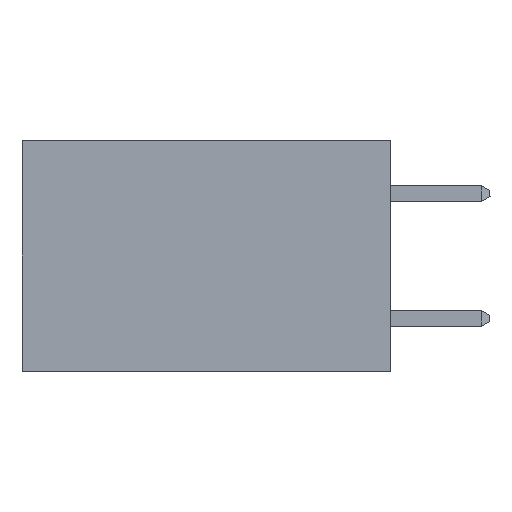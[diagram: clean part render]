
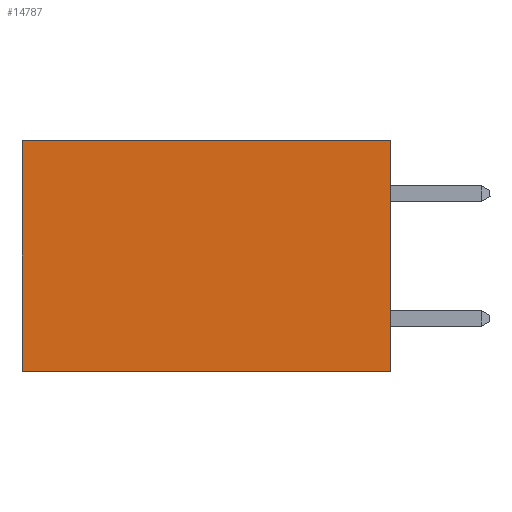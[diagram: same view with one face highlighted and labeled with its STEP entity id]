
A CAD part, left-side view. The second image highlights one B-rep face of the part: STEP entity #14787.
In plain terms, the highlighted planar face has unit normal (-1, 0, 0).
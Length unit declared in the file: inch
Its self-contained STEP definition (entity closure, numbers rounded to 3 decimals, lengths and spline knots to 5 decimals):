
#347 = CARTESIAN_POINT ( 'NONE',  ( 0.277, 0.59, 0. ) ) ;
#1477 = CARTESIAN_POINT ( 'NONE',  ( 0.277, 0., -0.37 ) ) ;
#1600 = CARTESIAN_POINT ( 'NONE',  ( 0.277, 0., -0.37 ) ) ;
#2965 = LINE ( 'NONE', #6803, #10829 ) ;
#3771 = ORIENTED_EDGE ( 'NONE', *, *, #13787, .F. ) ;
#4180 = AXIS2_PLACEMENT_3D ( 'NONE', #4374, #14548, #5916 ) ;
#4274 = FACE_OUTER_BOUND ( 'NONE', #13644, .T. ) ;
#4374 = CARTESIAN_POINT ( 'NONE',  ( 0.277, 0., -0.37 ) ) ;
#4384 = ORIENTED_EDGE ( 'NONE', *, *, #16679, .F. ) ;
#4889 = VECTOR ( 'NONE', #10450, 39.37008 ) ;
#5178 = CARTESIAN_POINT ( 'NONE',  ( 0.277, 0., 0. ) ) ;
#5480 = EDGE_CURVE ( 'NONE', #12283, #11610, #2965, .T. ) ;
#5916 = DIRECTION ( 'NONE',  ( 0., 0., -1. ) ) ;
#6198 = LINE ( 'NONE', #16697, #9669 ) ;
#6334 = ORIENTED_EDGE ( 'NONE', *, *, #15462, .T. ) ;
#6803 = CARTESIAN_POINT ( 'NONE',  ( 0.277, 0.59, -0.37 ) ) ;
#7529 = VECTOR ( 'NONE', #17961, 39.37008 ) ;
#9591 = CARTESIAN_POINT ( 'NONE',  ( 0.277, 0.59, -0.37 ) ) ;
#9669 = VECTOR ( 'NONE', #18142, 39.37008 ) ;
#9840 = DIRECTION ( 'NONE',  ( 0., 0., -1. ) ) ;
#10314 = PLANE ( 'NONE',  #4180 ) ;
#10450 = DIRECTION ( 'NONE',  ( 0., 0., -1. ) ) ;
#10829 = VECTOR ( 'NONE', #9840, 39.37008 ) ;
#11610 = VERTEX_POINT ( 'NONE', #9591 ) ;
#12237 = CARTESIAN_POINT ( 'NONE',  ( 0.277, 0., 0. ) ) ;
#12283 = VERTEX_POINT ( 'NONE', #347 ) ;
#12494 = ORIENTED_EDGE ( 'NONE', *, *, #5480, .T. ) ;
#12797 = VERTEX_POINT ( 'NONE', #1600 ) ;
#13644 = EDGE_LOOP ( 'NONE', ( #12494, #3771, #4384, #6334 ) ) ;
#13787 = EDGE_CURVE ( 'NONE', #12797, #11610, #6198, .T. ) ;
#14548 = DIRECTION ( 'NONE',  ( 1., 0., 0. ) ) ;
#14787 = ADVANCED_FACE ( 'NONE', ( #4274 ), #10314, .F. ) ;
#15129 = LINE ( 'NONE', #12237, #7529 ) ;
#15462 = EDGE_CURVE ( 'NONE', #17475, #12283, #15129, .T. ) ;
#15991 = LINE ( 'NONE', #1477, #4889 ) ;
#16679 = EDGE_CURVE ( 'NONE', #17475, #12797, #15991, .T. ) ;
#16697 = CARTESIAN_POINT ( 'NONE',  ( 0.277, 0., -0.37 ) ) ;
#17475 = VERTEX_POINT ( 'NONE', #5178 ) ;
#17961 = DIRECTION ( 'NONE',  ( 0., 1., 0. ) ) ;
#18142 = DIRECTION ( 'NONE',  ( 0., 1., 0. ) ) ;
